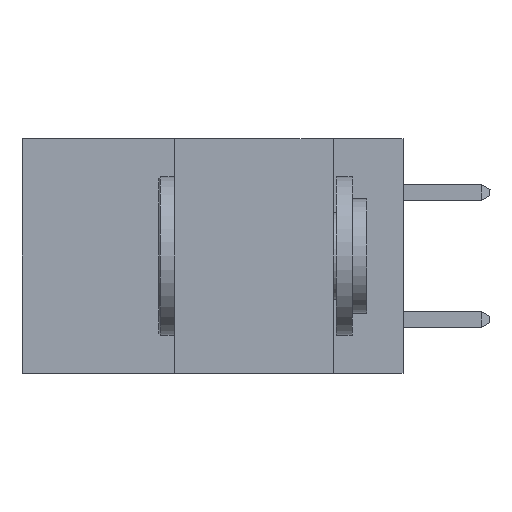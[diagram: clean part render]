
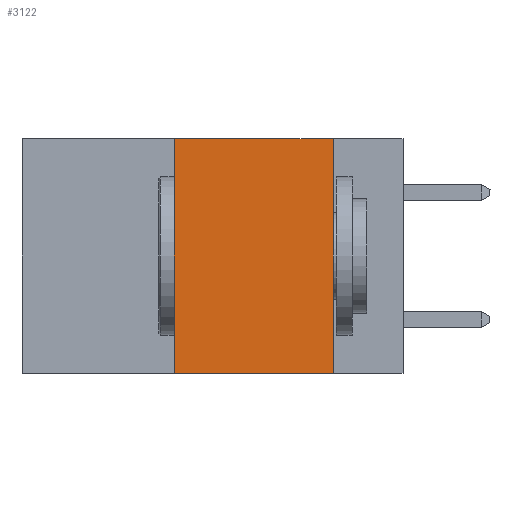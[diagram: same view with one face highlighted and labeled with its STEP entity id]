
A CAD part, left-side view. The second image highlights one B-rep face of the part: STEP entity #3122.
In plain terms, the highlighted planar face has unit normal (-1, 0, 0).
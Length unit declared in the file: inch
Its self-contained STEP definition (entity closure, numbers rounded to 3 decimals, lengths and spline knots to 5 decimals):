
#124 = VECTOR ( 'NONE', #3115, 39.37008 ) ;
#375 = LINE ( 'NONE', #31804, #9604 ) ;
#1550 = CARTESIAN_POINT ( 'NONE',  ( 0., 0.11, 0. ) ) ;
#2082 = ORIENTED_EDGE ( 'NONE', *, *, #32321, .T. ) ;
#2983 = DIRECTION ( 'NONE',  ( 0., 0., -1. ) ) ;
#3115 = DIRECTION ( 'NONE',  ( 0., -1., 0. ) ) ;
#3122 = ADVANCED_FACE ( 'NONE', ( #7598 ), #33607, .F. ) ;
#3207 = LINE ( 'NONE', #19940, #124 ) ;
#6408 = ORIENTED_EDGE ( 'NONE', *, *, #34800, .F. ) ;
#7598 = FACE_OUTER_BOUND ( 'NONE', #28745, .T. ) ;
#8074 = DIRECTION ( 'NONE',  ( 1., 0., 0. ) ) ;
#8186 = AXIS2_PLACEMENT_3D ( 'NONE', #20462, #8074, #8212 ) ;
#8212 = DIRECTION ( 'NONE',  ( 0., 0., -1. ) ) ;
#8483 = VERTEX_POINT ( 'NONE', #32255 ) ;
#9604 = VECTOR ( 'NONE', #26659, 39.37008 ) ;
#11337 = EDGE_CURVE ( 'NONE', #35672, #8483, #14780, .T. ) ;
#14713 = ORIENTED_EDGE ( 'NONE', *, *, #15828, .F. ) ;
#14780 = LINE ( 'NONE', #30856, #36366 ) ;
#15828 = EDGE_CURVE ( 'NONE', #32583, #28432, #32033, .T. ) ;
#16193 = VECTOR ( 'NONE', #31355, 39.37008 ) ;
#16316 = CARTESIAN_POINT ( 'NONE',  ( 0., 0.36, 0. ) ) ;
#19130 = CARTESIAN_POINT ( 'NONE',  ( 0., 0.36, 0. ) ) ;
#19940 = CARTESIAN_POINT ( 'NONE',  ( 0., 0.6, -0.37 ) ) ;
#20462 = CARTESIAN_POINT ( 'NONE',  ( 0., 0.6, 0. ) ) ;
#21279 = CARTESIAN_POINT ( 'NONE',  ( 0., 0.36, -0.37 ) ) ;
#26659 = DIRECTION ( 'NONE',  ( 0., -1., 0. ) ) ;
#27582 = ORIENTED_EDGE ( 'NONE', *, *, #11337, .F. ) ;
#28432 = VERTEX_POINT ( 'NONE', #16316 ) ;
#28745 = EDGE_LOOP ( 'NONE', ( #27582, #6408, #14713, #2082 ) ) ;
#30856 = CARTESIAN_POINT ( 'NONE',  ( 0., 0.11, 0. ) ) ;
#31355 = DIRECTION ( 'NONE',  ( 0., 0., 1. ) ) ;
#31804 = CARTESIAN_POINT ( 'NONE',  ( 0., 0.6, 0. ) ) ;
#32033 = LINE ( 'NONE', #19130, #16193 ) ;
#32255 = CARTESIAN_POINT ( 'NONE',  ( 0., 0.11, -0.37 ) ) ;
#32321 = EDGE_CURVE ( 'NONE', #32583, #8483, #3207, .T. ) ;
#32583 = VERTEX_POINT ( 'NONE', #21279 ) ;
#33607 = PLANE ( 'NONE',  #8186 ) ;
#34800 = EDGE_CURVE ( 'NONE', #28432, #35672, #375, .T. ) ;
#35672 = VERTEX_POINT ( 'NONE', #1550 ) ;
#36366 = VECTOR ( 'NONE', #2983, 39.37008 ) ;
